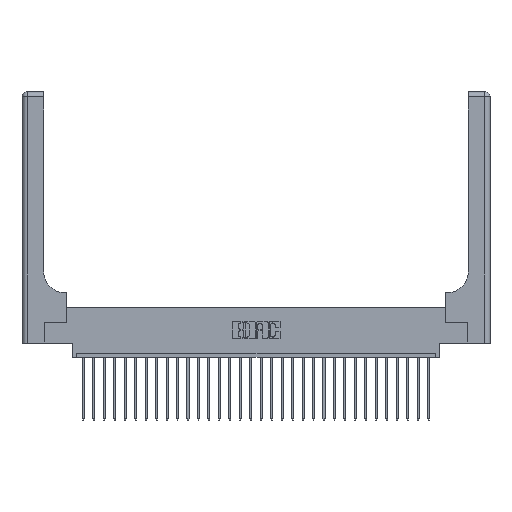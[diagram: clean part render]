
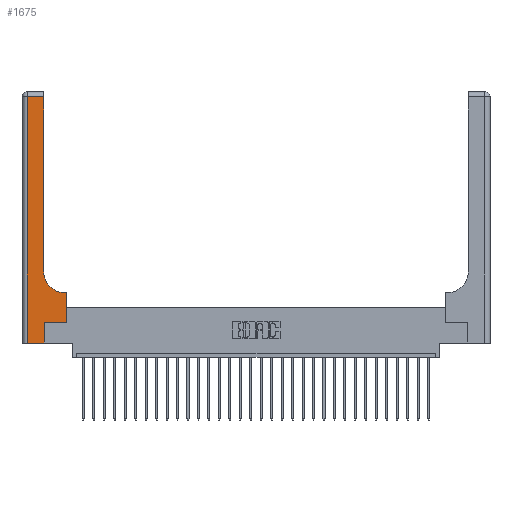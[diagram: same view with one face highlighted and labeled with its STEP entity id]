
A CAD part, top view. The second image highlights one B-rep face of the part: STEP entity #1675.
In plain terms, the highlighted planar face has unit normal (0, 0, 1).
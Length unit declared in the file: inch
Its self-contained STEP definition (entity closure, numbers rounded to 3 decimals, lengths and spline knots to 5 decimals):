
#44 = VECTOR ( 'NONE', #9920, 39.37008 ) ;
#161 = VERTEX_POINT ( 'NONE', #27315 ) ;
#297 = VERTEX_POINT ( 'NONE', #13289 ) ;
#362 = VERTEX_POINT ( 'NONE', #24438 ) ;
#950 = EDGE_CURVE ( 'NONE', #11667, #362, #1786, .T. ) ;
#1183 = CARTESIAN_POINT ( 'NONE',  ( 0.06, 2.94, 0.37 ) ) ;
#1437 = ORIENTED_EDGE ( 'NONE', *, *, #2780, .T. ) ;
#1675 = ADVANCED_FACE ( 'NONE', ( #23793 ), #25777, .F. ) ;
#1786 = LINE ( 'NONE', #19025, #22937 ) ;
#1894 = CARTESIAN_POINT ( 'NONE',  ( 0.528, 0.25, 0.37 ) ) ;
#2344 = AXIS2_PLACEMENT_3D ( 'NONE', #9279, #4876, #13358 ) ;
#2352 = ORIENTED_EDGE ( 'NONE', *, *, #20565, .T. ) ;
#2780 = EDGE_CURVE ( 'NONE', #6324, #297, #20846, .T. ) ;
#3284 = ORIENTED_EDGE ( 'NONE', *, *, #20855, .T. ) ;
#3690 = EDGE_CURVE ( 'NONE', #22266, #11667, #27009, .T. ) ;
#3959 = EDGE_CURVE ( 'NONE', #297, #25636, #18489, .T. ) ;
#4511 = ORIENTED_EDGE ( 'NONE', *, *, #3690, .T. ) ;
#4516 = EDGE_CURVE ( 'NONE', #25636, #18279, #4600, .T. ) ;
#4600 = CIRCLE ( 'NONE', #2344, 0.25 ) ;
#4876 = DIRECTION ( 'NONE',  ( 0., 0., -1. ) ) ;
#5990 = VECTOR ( 'NONE', #16890, 39.37008 ) ;
#6071 = VERTEX_POINT ( 'NONE', #1183 ) ;
#6324 = VERTEX_POINT ( 'NONE', #26620 ) ;
#6404 = VECTOR ( 'NONE', #17416, 39.37008 ) ;
#8285 = CARTESIAN_POINT ( 'NONE',  ( 0., 2.94, 0.37 ) ) ;
#9279 = CARTESIAN_POINT ( 'NONE',  ( 0.51, 0.85, 0.37 ) ) ;
#9715 = EDGE_LOOP ( 'NONE', ( #3284, #11182, #25624, #4511, #14794, #2352, #1437, #13233, #12223 ) ) ;
#9920 = DIRECTION ( 'NONE',  ( 1., 0., 0. ) ) ;
#11182 = ORIENTED_EDGE ( 'NONE', *, *, #23407, .T. ) ;
#11667 = VERTEX_POINT ( 'NONE', #22651 ) ;
#12223 = ORIENTED_EDGE ( 'NONE', *, *, #4516, .T. ) ;
#12565 = DIRECTION ( 'NONE',  ( 0., -1., 0. ) ) ;
#13233 = ORIENTED_EDGE ( 'NONE', *, *, #3959, .T. ) ;
#13289 = CARTESIAN_POINT ( 'NONE',  ( 0.528, 0.6, 0.37 ) ) ;
#13358 = DIRECTION ( 'NONE',  ( 1., 0., 0. ) ) ;
#13778 = CARTESIAN_POINT ( 'NONE',  ( 0.265, 0.25, 0.37 ) ) ;
#14794 = ORIENTED_EDGE ( 'NONE', *, *, #950, .T. ) ;
#14811 = AXIS2_PLACEMENT_3D ( 'NONE', #17012, #15165, #25638 ) ;
#14815 = CARTESIAN_POINT ( 'NONE',  ( 0.06, 3., 0.37 ) ) ;
#14893 = CARTESIAN_POINT ( 'NONE',  ( 0.26, 3., 0.37 ) ) ;
#15161 = LINE ( 'NONE', #14893, #6404 ) ;
#15165 = DIRECTION ( 'NONE',  ( 0., 0., -1. ) ) ;
#15745 = LINE ( 'NONE', #13778, #25806 ) ;
#16657 = CARTESIAN_POINT ( 'NONE',  ( 0.51, 0.6, 0.37 ) ) ;
#16890 = DIRECTION ( 'NONE',  ( -1., 0., 0. ) ) ;
#17012 = CARTESIAN_POINT ( 'NONE',  ( 0., 3., 0.37 ) ) ;
#17416 = DIRECTION ( 'NONE',  ( 0., 1., 0. ) ) ;
#17844 = VECTOR ( 'NONE', #12565, 39.37008 ) ;
#17869 = DIRECTION ( 'NONE',  ( 1., 0., 0. ) ) ;
#18279 = VERTEX_POINT ( 'NONE', #21144 ) ;
#18489 = LINE ( 'NONE', #25140, #27173 ) ;
#19008 = LINE ( 'NONE', #8285, #5990 ) ;
#19025 = CARTESIAN_POINT ( 'NONE',  ( 0.265, 0., 0.37 ) ) ;
#20565 = EDGE_CURVE ( 'NONE', #362, #6324, #15745, .T. ) ;
#20846 = LINE ( 'NONE', #1894, #27099 ) ;
#20855 = EDGE_CURVE ( 'NONE', #18279, #161, #15161, .T. ) ;
#21144 = CARTESIAN_POINT ( 'NONE',  ( 0.26, 0.85, 0.37 ) ) ;
#21267 = DIRECTION ( 'NONE',  ( 0., 1., 0. ) ) ;
#22266 = VERTEX_POINT ( 'NONE', #23354 ) ;
#22651 = CARTESIAN_POINT ( 'NONE',  ( 0.265, 0., 0.37 ) ) ;
#22937 = VECTOR ( 'NONE', #27383, 39.37008 ) ;
#23354 = CARTESIAN_POINT ( 'NONE',  ( 0.06, 0., 0.37 ) ) ;
#23407 = EDGE_CURVE ( 'NONE', #161, #6071, #19008, .T. ) ;
#23722 = LINE ( 'NONE', #14815, #17844 ) ;
#23793 = FACE_OUTER_BOUND ( 'NONE', #9715, .T. ) ;
#24438 = CARTESIAN_POINT ( 'NONE',  ( 0.265, 0.25, 0.37 ) ) ;
#25140 = CARTESIAN_POINT ( 'NONE',  ( 0.26, 0.6, 0.37 ) ) ;
#25624 = ORIENTED_EDGE ( 'NONE', *, *, #26942, .T. ) ;
#25636 = VERTEX_POINT ( 'NONE', #16657 ) ;
#25638 = DIRECTION ( 'NONE',  ( -1., 0., 0. ) ) ;
#25777 = PLANE ( 'NONE',  #14811 ) ;
#25806 = VECTOR ( 'NONE', #17869, 39.37008 ) ;
#26620 = CARTESIAN_POINT ( 'NONE',  ( 0.528, 0.25, 0.37 ) ) ;
#26875 = CARTESIAN_POINT ( 'NONE',  ( 0., 0., 0.37 ) ) ;
#26942 = EDGE_CURVE ( 'NONE', #6071, #22266, #23722, .T. ) ;
#27009 = LINE ( 'NONE', #26875, #44 ) ;
#27099 = VECTOR ( 'NONE', #21267, 39.37008 ) ;
#27129 = DIRECTION ( 'NONE',  ( -1., 0., 0. ) ) ;
#27173 = VECTOR ( 'NONE', #27129, 39.37008 ) ;
#27315 = CARTESIAN_POINT ( 'NONE',  ( 0.26, 2.94, 0.37 ) ) ;
#27383 = DIRECTION ( 'NONE',  ( 0., 1., 0. ) ) ;
